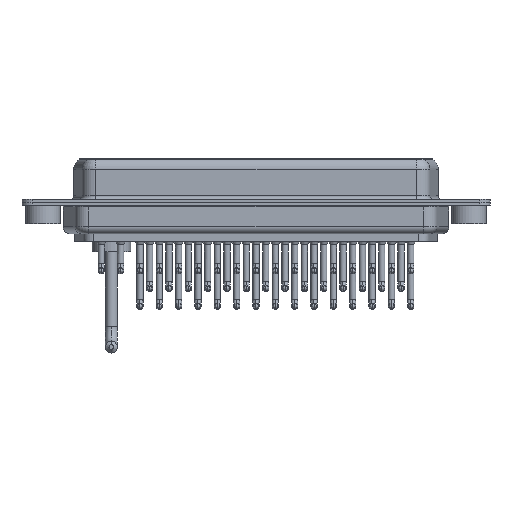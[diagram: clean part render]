
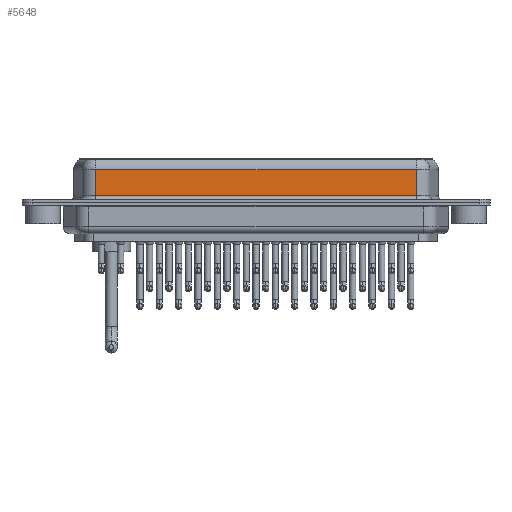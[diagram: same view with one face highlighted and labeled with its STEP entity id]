
A CAD part, front view. The second image highlights one B-rep face of the part: STEP entity #5648.
In plain terms, the highlighted planar face has unit normal (0, -1, 0).
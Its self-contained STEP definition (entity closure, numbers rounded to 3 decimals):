
#426 = LINE ( 'NONE', #13308, #25765 ) ;
#1060 = CARTESIAN_POINT ( 'NONE',  ( 53.41, -5.375, 6.4 ) ) ;
#1238 = FACE_OUTER_BOUND ( 'NONE', #1972, .T. ) ;
#1972 = EDGE_LOOP ( 'NONE', ( #13449, #3508, #23169, #26439 ) ) ;
#2153 = DIRECTION ( 'NONE',  ( 0., 0., -1. ) ) ;
#3508 = ORIENTED_EDGE ( 'NONE', *, *, #25068, .T. ) ;
#3539 = EDGE_CURVE ( 'NONE', #8743, #14106, #25157, .T. ) ;
#3623 = EDGE_CURVE ( 'NONE', #14106, #3934, #426, .T. ) ;
#3934 = VERTEX_POINT ( 'NONE', #17893 ) ;
#5648 = ADVANCED_FACE ( 'NONE', ( #1238 ), #16687, .F. ) ;
#6697 = VECTOR ( 'NONE', #18030, 1000. ) ;
#8415 = CARTESIAN_POINT ( 'NONE',  ( 7.59, -5.375, 4.65 ) ) ;
#8743 = VERTEX_POINT ( 'NONE', #8415 ) ;
#11172 = AXIS2_PLACEMENT_3D ( 'NONE', #1060, #11542, #16448 ) ;
#11542 = DIRECTION ( 'NONE',  ( 0., 1., 0. ) ) ;
#12227 = LINE ( 'NONE', #27998, #6697 ) ;
#13161 = VECTOR ( 'NONE', #14991, 1000. ) ;
#13308 = CARTESIAN_POINT ( 'NONE',  ( 53.41, -5.375, 0.9 ) ) ;
#13449 = ORIENTED_EDGE ( 'NONE', *, *, #26537, .F. ) ;
#14106 = VERTEX_POINT ( 'NONE', #28048 ) ;
#14991 = DIRECTION ( 'NONE',  ( -1., 0., 0. ) ) ;
#16448 = DIRECTION ( 'NONE',  ( 0., 0., 1. ) ) ;
#16687 = PLANE ( 'NONE',  #11172 ) ;
#17517 = VERTEX_POINT ( 'NONE', #30783 ) ;
#17893 = CARTESIAN_POINT ( 'NONE',  ( 53.41, -5.375, 0.9 ) ) ;
#18030 = DIRECTION ( 'NONE',  ( 0., 0., -1. ) ) ;
#22734 = CARTESIAN_POINT ( 'NONE',  ( 53.41, -5.375, 4.65 ) ) ;
#23169 = ORIENTED_EDGE ( 'NONE', *, *, #3539, .T. ) ;
#25068 = EDGE_CURVE ( 'NONE', #17517, #8743, #30621, .T. ) ;
#25157 = LINE ( 'NONE', #33392, #27985 ) ;
#25765 = VECTOR ( 'NONE', #31661, 1000. ) ;
#26439 = ORIENTED_EDGE ( 'NONE', *, *, #3623, .T. ) ;
#26537 = EDGE_CURVE ( 'NONE', #17517, #3934, #12227, .T. ) ;
#27985 = VECTOR ( 'NONE', #2153, 1000. ) ;
#27998 = CARTESIAN_POINT ( 'NONE',  ( 53.41, -5.375, 6.4 ) ) ;
#28048 = CARTESIAN_POINT ( 'NONE',  ( 7.59, -5.375, 0.9 ) ) ;
#30621 = LINE ( 'NONE', #22734, #13161 ) ;
#30783 = CARTESIAN_POINT ( 'NONE',  ( 53.41, -5.375, 4.65 ) ) ;
#31661 = DIRECTION ( 'NONE',  ( 1., 0., 0. ) ) ;
#33392 = CARTESIAN_POINT ( 'NONE',  ( 7.59, -5.375, 6.4 ) ) ;
